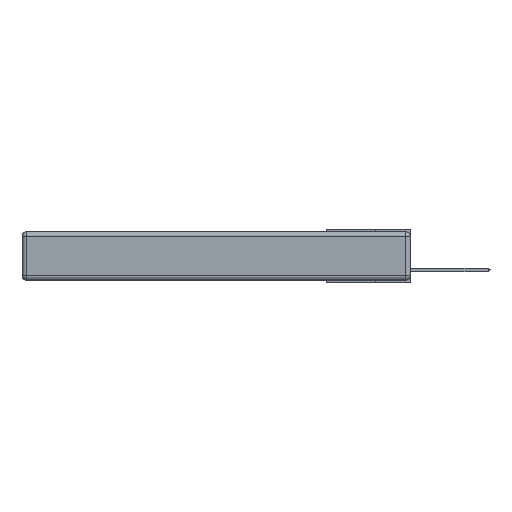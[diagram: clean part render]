
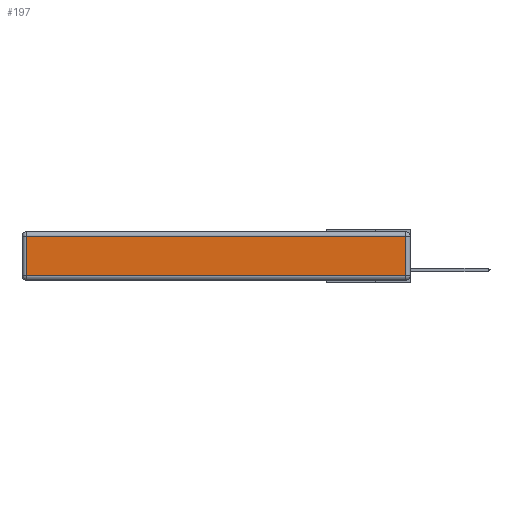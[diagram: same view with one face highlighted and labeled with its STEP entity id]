
A CAD part, left-side view. The second image highlights one B-rep face of the part: STEP entity #197.
In plain terms, the highlighted planar face has unit normal (-1, 0, 0).
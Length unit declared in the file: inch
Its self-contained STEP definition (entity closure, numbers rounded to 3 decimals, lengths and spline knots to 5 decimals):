
#197 = ADVANCED_FACE ( 'NONE', ( #2141 ), #22523, .T. ) ;
#204 = CARTESIAN_POINT ( 'NONE',  ( 0., 0.03, -0.313 ) ) ;
#1331 = DIRECTION ( 'NONE',  ( -1., 0., 0. ) ) ;
#2141 = FACE_OUTER_BOUND ( 'NONE', #8416, .T. ) ;
#4627 = DIRECTION ( 'NONE',  ( 0., 0., -1. ) ) ;
#4986 = CARTESIAN_POINT ( 'NONE',  ( 0., 0.03, -0.03 ) ) ;
#5674 = CARTESIAN_POINT ( 'NONE',  ( 0., 2.72, -0.03 ) ) ;
#6243 = CARTESIAN_POINT ( 'NONE',  ( 0., 0.03, -0.343 ) ) ;
#7025 = VECTOR ( 'NONE', #16904, 39.37008 ) ;
#7794 = VERTEX_POINT ( 'NONE', #4986 ) ;
#8416 = EDGE_LOOP ( 'NONE', ( #9717, #17499, #16002, #19318 ) ) ;
#9717 = ORIENTED_EDGE ( 'NONE', *, *, #12411, .T. ) ;
#10393 = EDGE_CURVE ( 'NONE', #7794, #15290, #19131, .T. ) ;
#10595 = DIRECTION ( 'NONE',  ( 0., 1., 0. ) ) ;
#10602 = LINE ( 'NONE', #17267, #16908 ) ;
#12411 = EDGE_CURVE ( 'NONE', #13284, #23666, #18298, .T. ) ;
#13284 = VERTEX_POINT ( 'NONE', #25758 ) ;
#13903 = CARTESIAN_POINT ( 'NONE',  ( 0., 0., -0.343 ) ) ;
#13991 = LINE ( 'NONE', #6243, #7025 ) ;
#15290 = VERTEX_POINT ( 'NONE', #5674 ) ;
#16002 = ORIENTED_EDGE ( 'NONE', *, *, #10393, .T. ) ;
#16030 = DIRECTION ( 'NONE',  ( 0., 0., 1. ) ) ;
#16300 = DIRECTION ( 'NONE',  ( 0., -1., 0. ) ) ;
#16904 = DIRECTION ( 'NONE',  ( 0., 0., 1. ) ) ;
#16908 = VECTOR ( 'NONE', #4627, 39.37008 ) ;
#17267 = CARTESIAN_POINT ( 'NONE',  ( 0., 2.72, -0.343 ) ) ;
#17499 = ORIENTED_EDGE ( 'NONE', *, *, #25475, .T. ) ;
#18298 = LINE ( 'NONE', #21129, #18661 ) ;
#18661 = VECTOR ( 'NONE', #16300, 39.37008 ) ;
#18789 = VECTOR ( 'NONE', #10595, 39.37008 ) ;
#19131 = LINE ( 'NONE', #23156, #18789 ) ;
#19318 = ORIENTED_EDGE ( 'NONE', *, *, #26769, .T. ) ;
#21129 = CARTESIAN_POINT ( 'NONE',  ( 0., 0., -0.313 ) ) ;
#22523 = PLANE ( 'NONE',  #24418 ) ;
#23156 = CARTESIAN_POINT ( 'NONE',  ( 0., 2.75, -0.03 ) ) ;
#23666 = VERTEX_POINT ( 'NONE', #204 ) ;
#24418 = AXIS2_PLACEMENT_3D ( 'NONE', #13903, #1331, #16030 ) ;
#25475 = EDGE_CURVE ( 'NONE', #23666, #7794, #13991, .T. ) ;
#25758 = CARTESIAN_POINT ( 'NONE',  ( 0., 2.72, -0.313 ) ) ;
#26769 = EDGE_CURVE ( 'NONE', #15290, #13284, #10602, .T. ) ;
